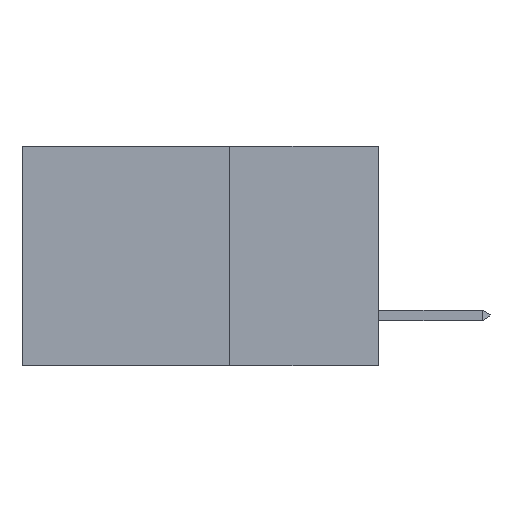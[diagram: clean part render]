
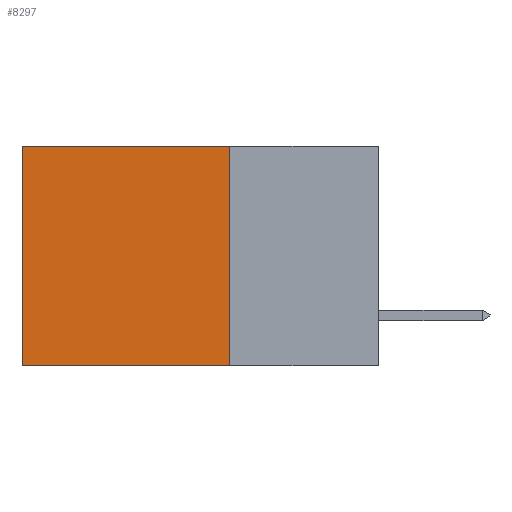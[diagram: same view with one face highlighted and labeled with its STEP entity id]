
A CAD part, left-side view. The second image highlights one B-rep face of the part: STEP entity #8297.
In plain terms, the highlighted planar face has unit normal (-1, 0, 0).
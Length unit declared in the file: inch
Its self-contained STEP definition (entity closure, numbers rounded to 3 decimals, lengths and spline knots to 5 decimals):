
#365 = LINE ( 'NONE', #1009, #2922 ) ;
#374 = VECTOR ( 'NONE', #4391, 39.37008 ) ;
#708 = CARTESIAN_POINT ( 'NONE',  ( 0.2615, 0.25, 0. ) ) ;
#730 = PLANE ( 'NONE',  #2339 ) ;
#1009 = CARTESIAN_POINT ( 'NONE',  ( 0.2615, 0.25, -0.37 ) ) ;
#1299 = ORIENTED_EDGE ( 'NONE', *, *, #11151, .F. ) ;
#2233 = VERTEX_POINT ( 'NONE', #7905 ) ;
#2339 = AXIS2_PLACEMENT_3D ( 'NONE', #10914, #4676, #3678 ) ;
#2623 = CARTESIAN_POINT ( 'NONE',  ( 0.2615, 0.25, 0. ) ) ;
#2922 = VECTOR ( 'NONE', #10317, 39.37008 ) ;
#3049 = CARTESIAN_POINT ( 'NONE',  ( 0.2615, 0.6, 0. ) ) ;
#3258 = VERTEX_POINT ( 'NONE', #2623 ) ;
#3364 = DIRECTION ( 'NONE',  ( 0., 0., -1. ) ) ;
#3464 = VERTEX_POINT ( 'NONE', #5000 ) ;
#3577 = ORIENTED_EDGE ( 'NONE', *, *, #4433, .T. ) ;
#3678 = DIRECTION ( 'NONE',  ( 0., 0., -1. ) ) ;
#4391 = DIRECTION ( 'NONE',  ( 0., 1., 0. ) ) ;
#4433 = EDGE_CURVE ( 'NONE', #3258, #5976, #6284, .T. ) ;
#4676 = DIRECTION ( 'NONE',  ( 1., 0., 0. ) ) ;
#5000 = CARTESIAN_POINT ( 'NONE',  ( 0.2615, 0.25, -0.37 ) ) ;
#5976 = VERTEX_POINT ( 'NONE', #3049 ) ;
#6284 = LINE ( 'NONE', #708, #374 ) ;
#7066 = DIRECTION ( 'NONE',  ( 0., 1., 0. ) ) ;
#7334 = EDGE_CURVE ( 'NONE', #5976, #2233, #7632, .T. ) ;
#7632 = LINE ( 'NONE', #11597, #9241 ) ;
#7905 = CARTESIAN_POINT ( 'NONE',  ( 0.2615, 0.6, -0.37 ) ) ;
#8297 = ADVANCED_FACE ( 'NONE', ( #9049 ), #730, .F. ) ;
#8375 = ORIENTED_EDGE ( 'NONE', *, *, #8673, .F. ) ;
#8673 = EDGE_CURVE ( 'NONE', #3464, #2233, #10066, .T. ) ;
#9049 = FACE_OUTER_BOUND ( 'NONE', #11135, .T. ) ;
#9241 = VECTOR ( 'NONE', #3364, 39.37008 ) ;
#10066 = LINE ( 'NONE', #10852, #10819 ) ;
#10317 = DIRECTION ( 'NONE',  ( 0., 0., -1. ) ) ;
#10376 = ORIENTED_EDGE ( 'NONE', *, *, #7334, .T. ) ;
#10819 = VECTOR ( 'NONE', #7066, 39.37008 ) ;
#10852 = CARTESIAN_POINT ( 'NONE',  ( 0.2615, 0.25, -0.37 ) ) ;
#10914 = CARTESIAN_POINT ( 'NONE',  ( 0.2615, 0.25, -0.37 ) ) ;
#11135 = EDGE_LOOP ( 'NONE', ( #10376, #8375, #1299, #3577 ) ) ;
#11151 = EDGE_CURVE ( 'NONE', #3258, #3464, #365, .T. ) ;
#11597 = CARTESIAN_POINT ( 'NONE',  ( 0.2615, 0.6, -0.37 ) ) ;
